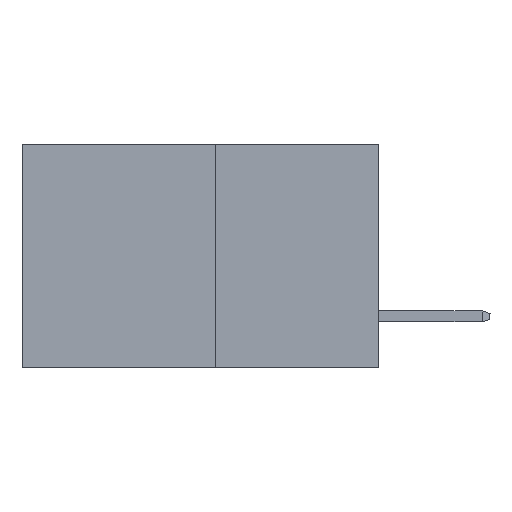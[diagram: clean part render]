
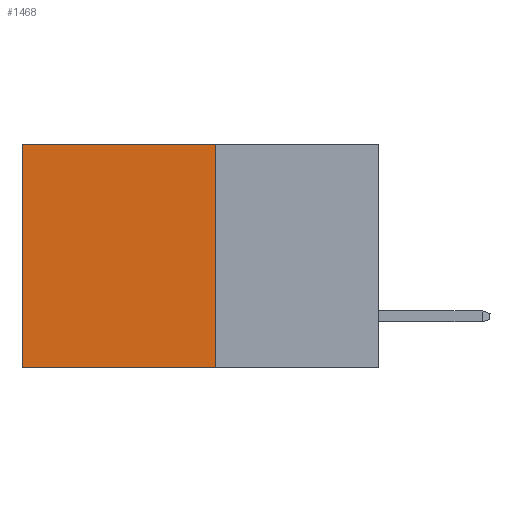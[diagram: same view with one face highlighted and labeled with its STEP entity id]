
A CAD part, left-side view. The second image highlights one B-rep face of the part: STEP entity #1468.
In plain terms, the highlighted planar face has unit normal (-1, 0, 0).
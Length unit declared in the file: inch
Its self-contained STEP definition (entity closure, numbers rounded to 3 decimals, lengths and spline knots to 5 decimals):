
#391 = FACE_OUTER_BOUND ( 'NONE', #13030, .T. ) ;
#504 = ORIENTED_EDGE ( 'NONE', *, *, #15742, .F. ) ;
#700 = VERTEX_POINT ( 'NONE', #23457 ) ;
#857 = VERTEX_POINT ( 'NONE', #13846 ) ;
#1468 = ADVANCED_FACE ( 'NONE', ( #391 ), #17562, .F. ) ;
#1806 = CARTESIAN_POINT ( 'NONE',  ( 0.277, 0.27, -0.37 ) ) ;
#3005 = LINE ( 'NONE', #22493, #25593 ) ;
#4787 = CARTESIAN_POINT ( 'NONE',  ( 0.277, 0.27, -0.37 ) ) ;
#5934 = LINE ( 'NONE', #1806, #29105 ) ;
#6117 = EDGE_CURVE ( 'NONE', #17828, #700, #23355, .T. ) ;
#6430 = CARTESIAN_POINT ( 'NONE',  ( 0.277, 0.59, -0.37 ) ) ;
#6989 = DIRECTION ( 'NONE',  ( 0., 0., -1. ) ) ;
#7041 = ORIENTED_EDGE ( 'NONE', *, *, #6117, .T. ) ;
#8008 = CARTESIAN_POINT ( 'NONE',  ( 0.277, 0.27, 0. ) ) ;
#9671 = EDGE_CURVE ( 'NONE', #17828, #857, #3005, .T. ) ;
#10343 = EDGE_CURVE ( 'NONE', #700, #18064, #13904, .T. ) ;
#10740 = ORIENTED_EDGE ( 'NONE', *, *, #9671, .F. ) ;
#11088 = AXIS2_PLACEMENT_3D ( 'NONE', #4787, #16948, #16857 ) ;
#11624 = DIRECTION ( 'NONE',  ( 0., 1., 0. ) ) ;
#13030 = EDGE_LOOP ( 'NONE', ( #14440, #504, #10740, #7041 ) ) ;
#13138 = DIRECTION ( 'NONE',  ( 0., 1., 0. ) ) ;
#13846 = CARTESIAN_POINT ( 'NONE',  ( 0.277, 0.27, -0.37 ) ) ;
#13904 = LINE ( 'NONE', #22770, #24505 ) ;
#14440 = ORIENTED_EDGE ( 'NONE', *, *, #10343, .T. ) ;
#15742 = EDGE_CURVE ( 'NONE', #857, #18064, #5934, .T. ) ;
#16100 = CARTESIAN_POINT ( 'NONE',  ( 0.277, 0.27, 0. ) ) ;
#16857 = DIRECTION ( 'NONE',  ( 0., 0., -1. ) ) ;
#16948 = DIRECTION ( 'NONE',  ( 1., 0., 0. ) ) ;
#17359 = VECTOR ( 'NONE', #11624, 39.37008 ) ;
#17562 = PLANE ( 'NONE',  #11088 ) ;
#17828 = VERTEX_POINT ( 'NONE', #8008 ) ;
#18064 = VERTEX_POINT ( 'NONE', #6430 ) ;
#22493 = CARTESIAN_POINT ( 'NONE',  ( 0.277, 0.27, -0.37 ) ) ;
#22770 = CARTESIAN_POINT ( 'NONE',  ( 0.277, 0.59, -0.37 ) ) ;
#23355 = LINE ( 'NONE', #16100, #17359 ) ;
#23457 = CARTESIAN_POINT ( 'NONE',  ( 0.277, 0.59, 0. ) ) ;
#24505 = VECTOR ( 'NONE', #6989, 39.37008 ) ;
#25593 = VECTOR ( 'NONE', #29196, 39.37008 ) ;
#29105 = VECTOR ( 'NONE', #13138, 39.37008 ) ;
#29196 = DIRECTION ( 'NONE',  ( 0., 0., -1. ) ) ;
